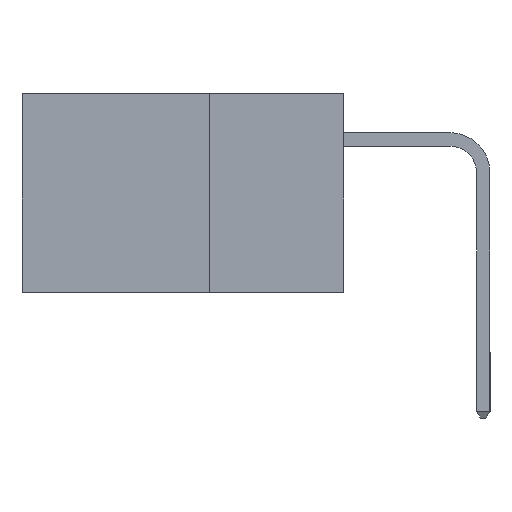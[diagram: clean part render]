
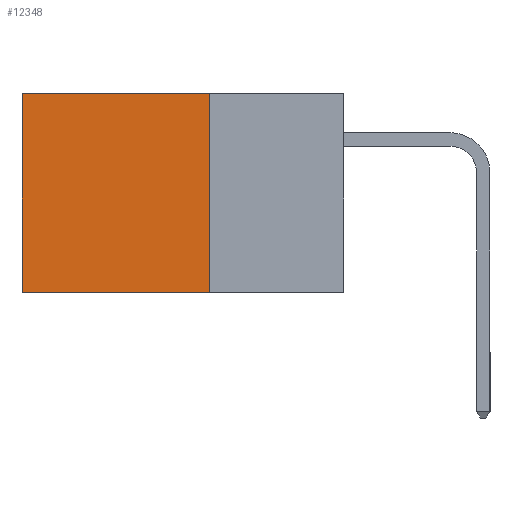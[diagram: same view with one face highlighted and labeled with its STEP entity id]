
A CAD part, left-side view. The second image highlights one B-rep face of the part: STEP entity #12348.
In plain terms, the highlighted planar face has unit normal (-1, 0, 0).
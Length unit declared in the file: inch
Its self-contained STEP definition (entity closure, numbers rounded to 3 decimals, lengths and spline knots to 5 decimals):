
#400 = CARTESIAN_POINT ( 'NONE',  ( 0.298, 0.6, -0.37 ) ) ;
#1559 = CARTESIAN_POINT ( 'NONE',  ( 0.298, 0.25, 0. ) ) ;
#2095 = VERTEX_POINT ( 'NONE', #10088 ) ;
#2147 = VECTOR ( 'NONE', #2710, 39.37008 ) ;
#2429 = EDGE_CURVE ( 'NONE', #2095, #10663, #7482, .T. ) ;
#2649 = VERTEX_POINT ( 'NONE', #12251 ) ;
#2710 = DIRECTION ( 'NONE',  ( 0., 0., -1. ) ) ;
#3102 = DIRECTION ( 'NONE',  ( 1., 0., 0. ) ) ;
#4342 = FACE_OUTER_BOUND ( 'NONE', #5106, .T. ) ;
#4466 = CARTESIAN_POINT ( 'NONE',  ( 0.298, 0.6, 0. ) ) ;
#4796 = CARTESIAN_POINT ( 'NONE',  ( 0.298, 0.25, 0. ) ) ;
#5106 = EDGE_LOOP ( 'NONE', ( #6136, #6159, #6695, #7003 ) ) ;
#6136 = ORIENTED_EDGE ( 'NONE', *, *, #10927, .T. ) ;
#6159 = ORIENTED_EDGE ( 'NONE', *, *, #2429, .F. ) ;
#6464 = EDGE_CURVE ( 'NONE', #7257, #2649, #6858, .T. ) ;
#6695 = ORIENTED_EDGE ( 'NONE', *, *, #13702, .F. ) ;
#6858 = LINE ( 'NONE', #4796, #12554 ) ;
#7003 = ORIENTED_EDGE ( 'NONE', *, *, #6464, .T. ) ;
#7176 = DIRECTION ( 'NONE',  ( 0., 1., 0. ) ) ;
#7257 = VERTEX_POINT ( 'NONE', #1559 ) ;
#7482 = LINE ( 'NONE', #10706, #12809 ) ;
#8670 = PLANE ( 'NONE',  #9446 ) ;
#9446 = AXIS2_PLACEMENT_3D ( 'NONE', #9753, #3102, #10807 ) ;
#9753 = CARTESIAN_POINT ( 'NONE',  ( 0.298, 0.25, 0. ) ) ;
#10088 = CARTESIAN_POINT ( 'NONE',  ( 0.298, 0.25, -0.37 ) ) ;
#10278 = VECTOR ( 'NONE', #12050, 39.37008 ) ;
#10430 = CARTESIAN_POINT ( 'NONE',  ( 0.298, 0.25, 0. ) ) ;
#10663 = VERTEX_POINT ( 'NONE', #400 ) ;
#10706 = CARTESIAN_POINT ( 'NONE',  ( 0.298, 0.25, -0.37 ) ) ;
#10748 = DIRECTION ( 'NONE',  ( 0., 1., 0. ) ) ;
#10807 = DIRECTION ( 'NONE',  ( 0., 0., -1. ) ) ;
#10927 = EDGE_CURVE ( 'NONE', #2649, #10663, #13029, .T. ) ;
#10963 = LINE ( 'NONE', #10430, #2147 ) ;
#12050 = DIRECTION ( 'NONE',  ( 0., 0., -1. ) ) ;
#12251 = CARTESIAN_POINT ( 'NONE',  ( 0.298, 0.6, 0. ) ) ;
#12348 = ADVANCED_FACE ( 'NONE', ( #4342 ), #8670, .F. ) ;
#12554 = VECTOR ( 'NONE', #7176, 39.37008 ) ;
#12809 = VECTOR ( 'NONE', #10748, 39.37008 ) ;
#13029 = LINE ( 'NONE', #4466, #10278 ) ;
#13702 = EDGE_CURVE ( 'NONE', #7257, #2095, #10963, .T. ) ;
